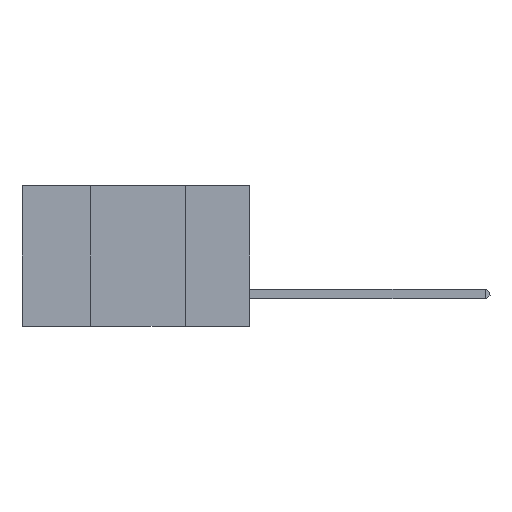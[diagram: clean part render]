
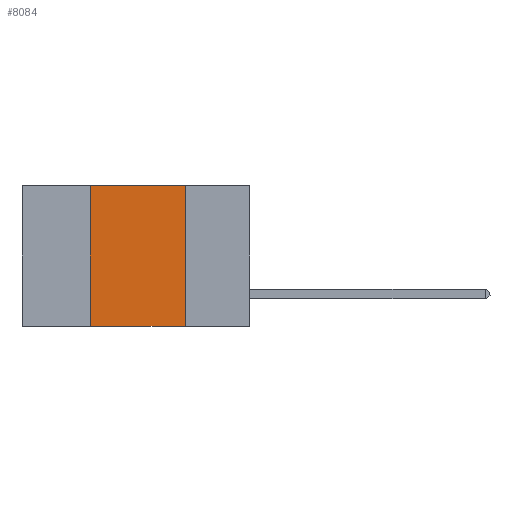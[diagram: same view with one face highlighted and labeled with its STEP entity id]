
A CAD part, left-side view. The second image highlights one B-rep face of the part: STEP entity #8084.
In plain terms, the highlighted planar face has unit normal (-1, 0, 0).
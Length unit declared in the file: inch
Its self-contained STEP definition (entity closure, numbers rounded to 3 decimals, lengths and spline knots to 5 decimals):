
#272 = EDGE_CURVE ( 'NONE', #12252, #2732, #8386, .T. ) ;
#389 = CARTESIAN_POINT ( 'NONE',  ( 0., 0.17, 0. ) ) ;
#783 = VECTOR ( 'NONE', #2669, 39.37008 ) ;
#986 = VERTEX_POINT ( 'NONE', #6147 ) ;
#1235 = CARTESIAN_POINT ( 'NONE',  ( 0., 0.17, 0. ) ) ;
#1880 = ORIENTED_EDGE ( 'NONE', *, *, #11095, .T. ) ;
#1923 = CARTESIAN_POINT ( 'NONE',  ( 0., 0.6, 0. ) ) ;
#1997 = VECTOR ( 'NONE', #10049, 39.37008 ) ;
#2300 = EDGE_CURVE ( 'NONE', #5998, #986, #7988, .T. ) ;
#2669 = DIRECTION ( 'NONE',  ( 0., -1., 0. ) ) ;
#2732 = VERTEX_POINT ( 'NONE', #5114 ) ;
#2735 = VECTOR ( 'NONE', #6337, 39.37008 ) ;
#3559 = DIRECTION ( 'NONE',  ( 1., 0., 0. ) ) ;
#4101 = EDGE_LOOP ( 'NONE', ( #9393, #6815, #12657, #1880 ) ) ;
#5114 = CARTESIAN_POINT ( 'NONE',  ( 0., 0.42, 0. ) ) ;
#5115 = EDGE_CURVE ( 'NONE', #2732, #5998, #7120, .T. ) ;
#5647 = VECTOR ( 'NONE', #8357, 39.37008 ) ;
#5998 = VERTEX_POINT ( 'NONE', #389 ) ;
#6147 = CARTESIAN_POINT ( 'NONE',  ( 0., 0.17, -0.37 ) ) ;
#6313 = CARTESIAN_POINT ( 'NONE',  ( 0., 0.42, 0. ) ) ;
#6337 = DIRECTION ( 'NONE',  ( 0., 0., -1. ) ) ;
#6815 = ORIENTED_EDGE ( 'NONE', *, *, #5115, .F. ) ;
#7017 = LINE ( 'NONE', #10909, #783 ) ;
#7120 = LINE ( 'NONE', #1923, #1997 ) ;
#7988 = LINE ( 'NONE', #1235, #2735 ) ;
#8084 = ADVANCED_FACE ( 'NONE', ( #11382 ), #12124, .F. ) ;
#8357 = DIRECTION ( 'NONE',  ( 0., 0., 1. ) ) ;
#8386 = LINE ( 'NONE', #6313, #5647 ) ;
#9393 = ORIENTED_EDGE ( 'NONE', *, *, #2300, .F. ) ;
#9399 = AXIS2_PLACEMENT_3D ( 'NONE', #9646, #3559, #11814 ) ;
#9646 = CARTESIAN_POINT ( 'NONE',  ( 0., 0.6, 0. ) ) ;
#10049 = DIRECTION ( 'NONE',  ( 0., -1., 0. ) ) ;
#10909 = CARTESIAN_POINT ( 'NONE',  ( 0., 0.6, -0.37 ) ) ;
#11095 = EDGE_CURVE ( 'NONE', #12252, #986, #7017, .T. ) ;
#11382 = FACE_OUTER_BOUND ( 'NONE', #4101, .T. ) ;
#11769 = CARTESIAN_POINT ( 'NONE',  ( 0., 0.42, -0.37 ) ) ;
#11814 = DIRECTION ( 'NONE',  ( 0., 0., -1. ) ) ;
#12124 = PLANE ( 'NONE',  #9399 ) ;
#12252 = VERTEX_POINT ( 'NONE', #11769 ) ;
#12657 = ORIENTED_EDGE ( 'NONE', *, *, #272, .F. ) ;
